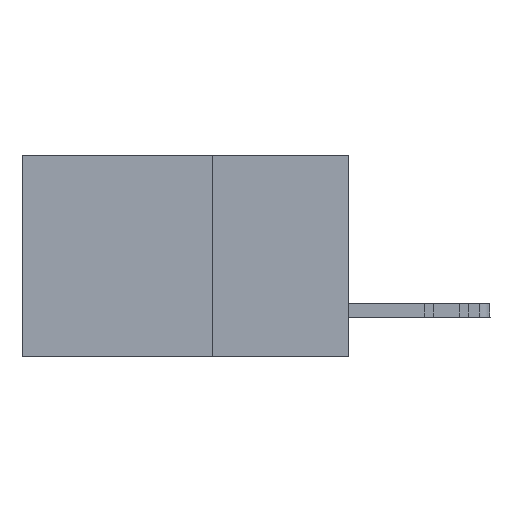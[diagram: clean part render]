
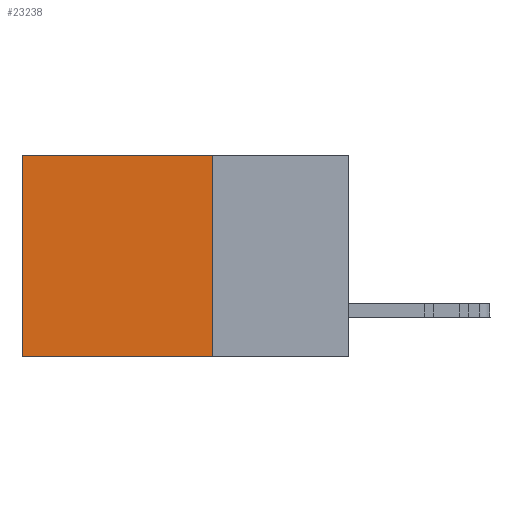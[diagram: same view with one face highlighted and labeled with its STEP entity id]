
A CAD part, left-side view. The second image highlights one B-rep face of the part: STEP entity #23238.
In plain terms, the highlighted planar face has unit normal (-1, 0, 0).
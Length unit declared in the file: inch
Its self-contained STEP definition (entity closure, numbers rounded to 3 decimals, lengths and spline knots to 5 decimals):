
#475 = CARTESIAN_POINT ( 'NONE',  ( 0.298, 0.6, -0.37 ) ) ;
#1021 = LINE ( 'NONE', #7667, #8830 ) ;
#2611 = VERTEX_POINT ( 'NONE', #3858 ) ;
#3858 = CARTESIAN_POINT ( 'NONE',  ( 0.298, 0.25, 0. ) ) ;
#4742 = DIRECTION ( 'NONE',  ( 0., 1., 0. ) ) ;
#5417 = DIRECTION ( 'NONE',  ( 0., 0., -1. ) ) ;
#6512 = LINE ( 'NONE', #8781, #18501 ) ;
#7167 = LINE ( 'NONE', #23301, #28518 ) ;
#7667 = CARTESIAN_POINT ( 'NONE',  ( 0.298, 0.25, -0.37 ) ) ;
#8781 = CARTESIAN_POINT ( 'NONE',  ( 0.298, 0.6, 0. ) ) ;
#8830 = VECTOR ( 'NONE', #10406, 39.37008 ) ;
#9182 = VERTEX_POINT ( 'NONE', #475 ) ;
#9554 = ORIENTED_EDGE ( 'NONE', *, *, #21380, .F. ) ;
#9593 = VERTEX_POINT ( 'NONE', #28494 ) ;
#9995 = ORIENTED_EDGE ( 'NONE', *, *, #23330, .T. ) ;
#10225 = EDGE_LOOP ( 'NONE', ( #10526, #9554, #27271, #9995 ) ) ;
#10406 = DIRECTION ( 'NONE',  ( 0., 1., 0. ) ) ;
#10526 = ORIENTED_EDGE ( 'NONE', *, *, #18301, .T. ) ;
#10893 = DIRECTION ( 'NONE',  ( 0., 0., -1. ) ) ;
#11224 = EDGE_CURVE ( 'NONE', #2611, #12655, #28024, .T. ) ;
#12655 = VERTEX_POINT ( 'NONE', #22176 ) ;
#15530 = FACE_OUTER_BOUND ( 'NONE', #10225, .T. ) ;
#16956 = CARTESIAN_POINT ( 'NONE',  ( 0.298, 0.25, 0. ) ) ;
#17688 = PLANE ( 'NONE',  #18869 ) ;
#18301 = EDGE_CURVE ( 'NONE', #9593, #9182, #6512, .T. ) ;
#18501 = VECTOR ( 'NONE', #10893, 39.37008 ) ;
#18869 = AXIS2_PLACEMENT_3D ( 'NONE', #24831, #27241, #22878 ) ;
#21380 = EDGE_CURVE ( 'NONE', #12655, #9182, #1021, .T. ) ;
#21402 = VECTOR ( 'NONE', #5417, 39.37008 ) ;
#22176 = CARTESIAN_POINT ( 'NONE',  ( 0.298, 0.25, -0.37 ) ) ;
#22878 = DIRECTION ( 'NONE',  ( 0., 0., -1. ) ) ;
#23238 = ADVANCED_FACE ( 'NONE', ( #15530 ), #17688, .F. ) ;
#23301 = CARTESIAN_POINT ( 'NONE',  ( 0.298, 0.25, 0. ) ) ;
#23330 = EDGE_CURVE ( 'NONE', #2611, #9593, #7167, .T. ) ;
#24831 = CARTESIAN_POINT ( 'NONE',  ( 0.298, 0.25, 0. ) ) ;
#27241 = DIRECTION ( 'NONE',  ( 1., 0., 0. ) ) ;
#27271 = ORIENTED_EDGE ( 'NONE', *, *, #11224, .F. ) ;
#28024 = LINE ( 'NONE', #16956, #21402 ) ;
#28494 = CARTESIAN_POINT ( 'NONE',  ( 0.298, 0.6, 0. ) ) ;
#28518 = VECTOR ( 'NONE', #4742, 39.37008 ) ;
